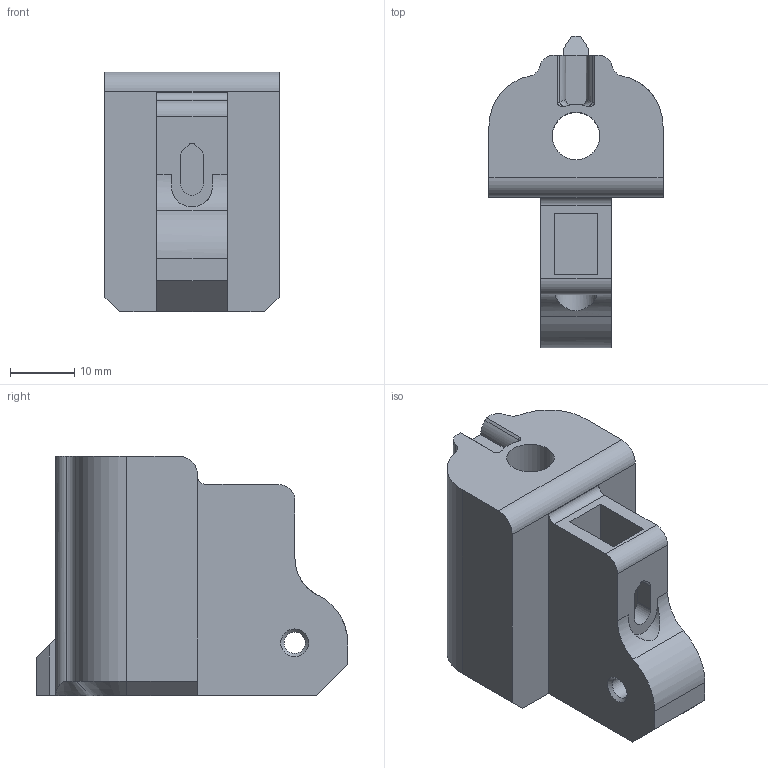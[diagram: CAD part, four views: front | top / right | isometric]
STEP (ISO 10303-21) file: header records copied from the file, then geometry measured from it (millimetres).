
FILE_DESCRIPTION(/* description */ ('STEP AP242','CAx-IF Rec.Pracs.---Representation and Presentation of Product Manufacturing Information (PMI)---4.0---2014-10-13','CAx-IF Rec.Pracs.---3D Tessellated Geometry---0.4---2014-09-14','2;1'),/* implementation_level */ '2;1');
FILE_NAME(/* name */ '61f05eaaccc8b87296449b06',/* time_stamp */ '2022-01-25T20:33:46+00:00',/* author */ (''),/* organization */ (''),/* preprocessor_version */ 'ST-DEVELOPER v18.101',/* originating_system */ ' ',/* authorisation */ ' ');
FILE_SCHEMA (('AP242_MANAGED_MODEL_BASED_3D_ENGINEERING_MIM_LF { 1 0 10303 442 1 1 4 }'));
Length unit declared in the file: metre
Products named in the file (1): Snub Barrel mk4
Bounding box: 27 x 48.29 x 37.18 mm (x, y, z)
Volume: 21780.1 mm3; surface area: 7964.5 mm2
Topology: 1 solids, 1 shells, 160 faces, 447 edges, 297 vertices
Faces by surface type: plane 72, bspline 51, cylinder 31, cone 6
Full cylindrical faces by diameter (mm): 3.302 x1, 7.366 x1
Entity records: 5546 total; most frequent: CARTESIAN_POINT 1828, ORIENTED_EDGE 884, DIRECTION 573, EDGE_CURVE 442, VERTEX_POINT 296, LINE 193, VECTOR 193, AXIS2_PLACEMENT_3D 190
